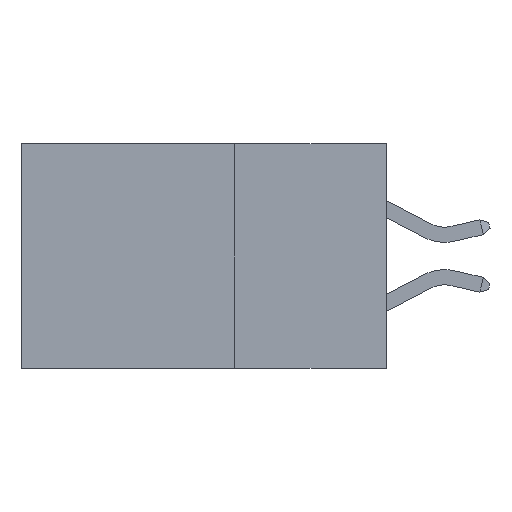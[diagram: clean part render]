
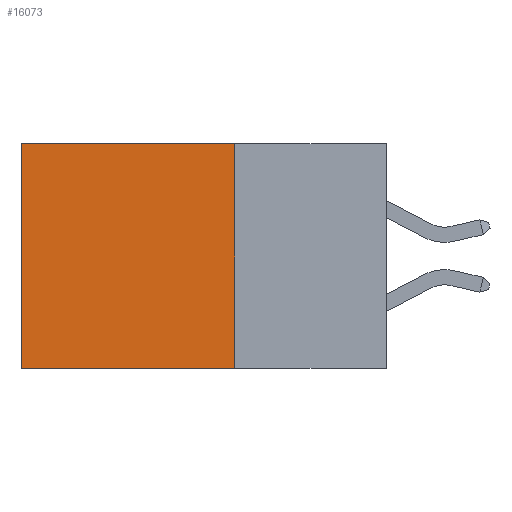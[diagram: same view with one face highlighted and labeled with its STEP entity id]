
A CAD part, left-side view. The second image highlights one B-rep face of the part: STEP entity #16073.
In plain terms, the highlighted planar face has unit normal (-1, 0, 0).
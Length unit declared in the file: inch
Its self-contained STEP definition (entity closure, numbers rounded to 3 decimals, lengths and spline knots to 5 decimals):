
#604 = VERTEX_POINT ( 'NONE', #12870 ) ;
#1644 = CARTESIAN_POINT ( 'NONE',  ( 0.2615, 0.25, 0. ) ) ;
#2062 = VERTEX_POINT ( 'NONE', #12969 ) ;
#2682 = ORIENTED_EDGE ( 'NONE', *, *, #8052, .T. ) ;
#3513 = VECTOR ( 'NONE', #8176, 39.37008 ) ;
#3552 = EDGE_LOOP ( 'NONE', ( #7837, #6677, #4780, #2682 ) ) ;
#3869 = LINE ( 'NONE', #12896, #4798 ) ;
#4115 = VERTEX_POINT ( 'NONE', #14345 ) ;
#4117 = LINE ( 'NONE', #1644, #14590 ) ;
#4140 = EDGE_CURVE ( 'NONE', #604, #2062, #3869, .T. ) ;
#4780 = ORIENTED_EDGE ( 'NONE', *, *, #4140, .F. ) ;
#4798 = VECTOR ( 'NONE', #6544, 39.37008 ) ;
#4888 = VERTEX_POINT ( 'NONE', #16410 ) ;
#6544 = DIRECTION ( 'NONE',  ( 0., 0., -1. ) ) ;
#6677 = ORIENTED_EDGE ( 'NONE', *, *, #14439, .F. ) ;
#6980 = EDGE_CURVE ( 'NONE', #4888, #4115, #16282, .T. ) ;
#7229 = PLANE ( 'NONE',  #9182 ) ;
#7837 = ORIENTED_EDGE ( 'NONE', *, *, #6980, .T. ) ;
#7994 = CARTESIAN_POINT ( 'NONE',  ( 0.2615, 0.25, -0.37 ) ) ;
#8052 = EDGE_CURVE ( 'NONE', #604, #4888, #4117, .T. ) ;
#8176 = DIRECTION ( 'NONE',  ( 0., 0., -1. ) ) ;
#8493 = CARTESIAN_POINT ( 'NONE',  ( 0.2615, 0.25, -0.37 ) ) ;
#9182 = AXIS2_PLACEMENT_3D ( 'NONE', #8493, #12634, #11106 ) ;
#9881 = FACE_OUTER_BOUND ( 'NONE', #3552, .T. ) ;
#11106 = DIRECTION ( 'NONE',  ( 0., 0., -1. ) ) ;
#12634 = DIRECTION ( 'NONE',  ( 1., 0., 0. ) ) ;
#12870 = CARTESIAN_POINT ( 'NONE',  ( 0.2615, 0.25, 0. ) ) ;
#12896 = CARTESIAN_POINT ( 'NONE',  ( 0.2615, 0.25, -0.37 ) ) ;
#12969 = CARTESIAN_POINT ( 'NONE',  ( 0.2615, 0.25, -0.37 ) ) ;
#14345 = CARTESIAN_POINT ( 'NONE',  ( 0.2615, 0.6, -0.37 ) ) ;
#14439 = EDGE_CURVE ( 'NONE', #2062, #4115, #15752, .T. ) ;
#14590 = VECTOR ( 'NONE', #14601, 39.37008 ) ;
#14601 = DIRECTION ( 'NONE',  ( 0., 1., 0. ) ) ;
#14697 = DIRECTION ( 'NONE',  ( 0., 1., 0. ) ) ;
#15064 = CARTESIAN_POINT ( 'NONE',  ( 0.2615, 0.6, -0.37 ) ) ;
#15740 = VECTOR ( 'NONE', #14697, 39.37008 ) ;
#15752 = LINE ( 'NONE', #7994, #15740 ) ;
#16073 = ADVANCED_FACE ( 'NONE', ( #9881 ), #7229, .F. ) ;
#16282 = LINE ( 'NONE', #15064, #3513 ) ;
#16410 = CARTESIAN_POINT ( 'NONE',  ( 0.2615, 0.6, 0. ) ) ;
